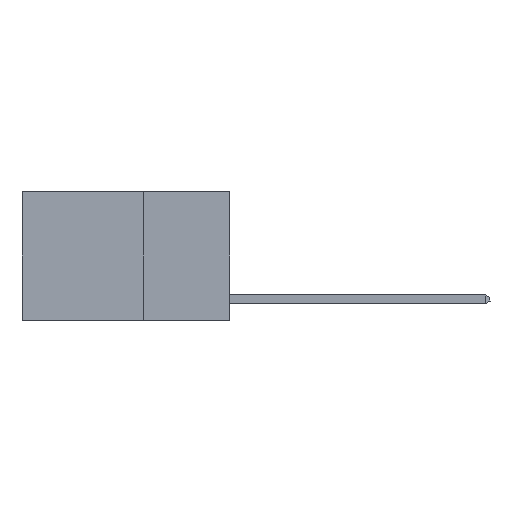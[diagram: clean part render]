
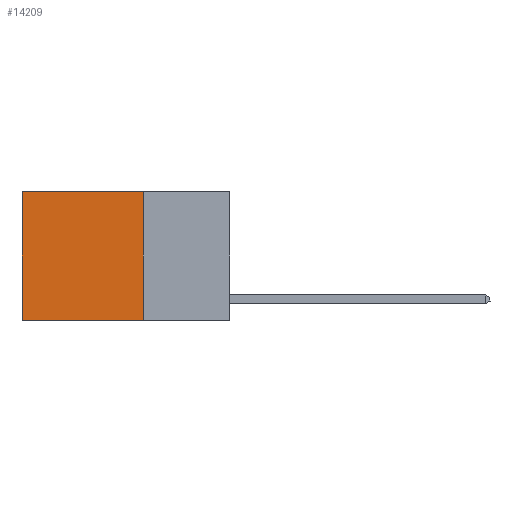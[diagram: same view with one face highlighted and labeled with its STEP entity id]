
A CAD part, left-side view. The second image highlights one B-rep face of the part: STEP entity #14209.
In plain terms, the highlighted planar face has unit normal (-1, 0, 0).
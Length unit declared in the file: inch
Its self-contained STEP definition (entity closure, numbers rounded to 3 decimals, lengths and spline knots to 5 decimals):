
#574 = DIRECTION ( 'NONE',  ( 0., 1., 0. ) ) ;
#1054 = CARTESIAN_POINT ( 'NONE',  ( 0.2625, 0.25, 0. ) ) ;
#1373 = VERTEX_POINT ( 'NONE', #2706 ) ;
#1447 = ORIENTED_EDGE ( 'NONE', *, *, #7837, .T. ) ;
#1466 = LINE ( 'NONE', #18386, #21229 ) ;
#1468 = DIRECTION ( 'NONE',  ( 1., 0., 0. ) ) ;
#2390 = EDGE_CURVE ( 'NONE', #10757, #19252, #18543, .T. ) ;
#2706 = CARTESIAN_POINT ( 'NONE',  ( 0.2625, 0.25, 0. ) ) ;
#3322 = DIRECTION ( 'NONE',  ( 0., 0., -1. ) ) ;
#4116 = LINE ( 'NONE', #15900, #17395 ) ;
#5699 = DIRECTION ( 'NONE',  ( 0., 1., 0. ) ) ;
#6212 = CARTESIAN_POINT ( 'NONE',  ( 0.2625, 0.6, -0.37 ) ) ;
#7281 = ORIENTED_EDGE ( 'NONE', *, *, #2390, .F. ) ;
#7494 = LINE ( 'NONE', #1054, #11756 ) ;
#7837 = EDGE_CURVE ( 'NONE', #14212, #19252, #4116, .T. ) ;
#8259 = EDGE_LOOP ( 'NONE', ( #1447, #7281, #22354, #13458 ) ) ;
#8385 = DIRECTION ( 'NONE',  ( 0., 0., -1. ) ) ;
#8999 = VECTOR ( 'NONE', #574, 39.37008 ) ;
#9240 = FACE_OUTER_BOUND ( 'NONE', #8259, .T. ) ;
#10757 = VERTEX_POINT ( 'NONE', #15610 ) ;
#11756 = VECTOR ( 'NONE', #8385, 39.37008 ) ;
#13458 = ORIENTED_EDGE ( 'NONE', *, *, #21579, .T. ) ;
#14066 = CARTESIAN_POINT ( 'NONE',  ( 0.2625, 0.25, 0. ) ) ;
#14136 = DIRECTION ( 'NONE',  ( 0., 0., -1. ) ) ;
#14209 = ADVANCED_FACE ( 'NONE', ( #9240 ), #23110, .F. ) ;
#14212 = VERTEX_POINT ( 'NONE', #21271 ) ;
#14774 = EDGE_CURVE ( 'NONE', #1373, #10757, #7494, .T. ) ;
#15394 = AXIS2_PLACEMENT_3D ( 'NONE', #14066, #1468, #14136 ) ;
#15610 = CARTESIAN_POINT ( 'NONE',  ( 0.2625, 0.25, -0.37 ) ) ;
#15900 = CARTESIAN_POINT ( 'NONE',  ( 0.2625, 0.6, 0. ) ) ;
#17395 = VECTOR ( 'NONE', #3322, 39.37008 ) ;
#18386 = CARTESIAN_POINT ( 'NONE',  ( 0.2625, 0.25, 0. ) ) ;
#18543 = LINE ( 'NONE', #22177, #8999 ) ;
#19252 = VERTEX_POINT ( 'NONE', #6212 ) ;
#21229 = VECTOR ( 'NONE', #5699, 39.37008 ) ;
#21271 = CARTESIAN_POINT ( 'NONE',  ( 0.2625, 0.6, 0. ) ) ;
#21579 = EDGE_CURVE ( 'NONE', #1373, #14212, #1466, .T. ) ;
#22177 = CARTESIAN_POINT ( 'NONE',  ( 0.2625, 0.25, -0.37 ) ) ;
#22354 = ORIENTED_EDGE ( 'NONE', *, *, #14774, .F. ) ;
#23110 = PLANE ( 'NONE',  #15394 ) ;
